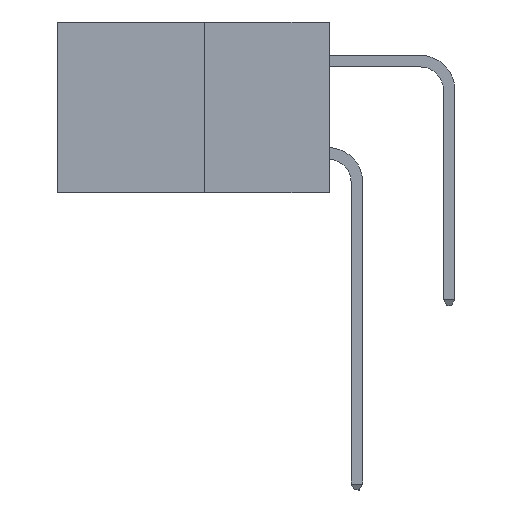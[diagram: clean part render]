
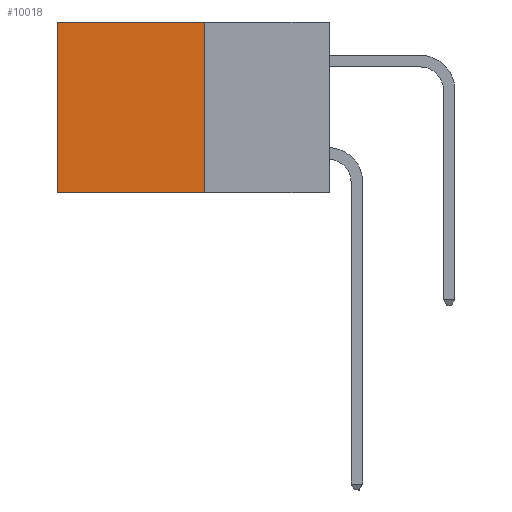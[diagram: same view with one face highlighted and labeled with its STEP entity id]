
A CAD part, left-side view. The second image highlights one B-rep face of the part: STEP entity #10018.
In plain terms, the highlighted planar face has unit normal (-1, 0, 0).
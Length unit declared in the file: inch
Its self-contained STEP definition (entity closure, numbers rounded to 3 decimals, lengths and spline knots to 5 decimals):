
#213 = ORIENTED_EDGE ( 'NONE', *, *, #5932, .T. ) ;
#272 = VECTOR ( 'NONE', #13073, 39.37008 ) ;
#283 = ORIENTED_EDGE ( 'NONE', *, *, #8095, .F. ) ;
#650 = VERTEX_POINT ( 'NONE', #18060 ) ;
#937 = ORIENTED_EDGE ( 'NONE', *, *, #4957, .F. ) ;
#2012 = VECTOR ( 'NONE', #16059, 39.37008 ) ;
#2642 = ORIENTED_EDGE ( 'NONE', *, *, #15275, .T. ) ;
#2751 = FACE_OUTER_BOUND ( 'NONE', #8653, .T. ) ;
#2906 = CARTESIAN_POINT ( 'NONE',  ( 0.277, 0.27, 0. ) ) ;
#4400 = PLANE ( 'NONE',  #9622 ) ;
#4454 = DIRECTION ( 'NONE',  ( 0., 0., -1. ) ) ;
#4722 = CARTESIAN_POINT ( 'NONE',  ( 0.277, 0.59, -0.37 ) ) ;
#4957 = EDGE_CURVE ( 'NONE', #17669, #8572, #16429, .T. ) ;
#5798 = DIRECTION ( 'NONE',  ( 0., 0., -1. ) ) ;
#5932 = EDGE_CURVE ( 'NONE', #11860, #650, #10958, .T. ) ;
#8095 = EDGE_CURVE ( 'NONE', #11860, #17669, #15264, .T. ) ;
#8271 = VECTOR ( 'NONE', #4454, 39.37008 ) ;
#8572 = VERTEX_POINT ( 'NONE', #17896 ) ;
#8653 = EDGE_LOOP ( 'NONE', ( #2642, #937, #283, #213 ) ) ;
#9010 = LINE ( 'NONE', #4722, #272 ) ;
#9176 = CARTESIAN_POINT ( 'NONE',  ( 0.277, 0.27, 0. ) ) ;
#9622 = AXIS2_PLACEMENT_3D ( 'NONE', #16898, #14138, #5798 ) ;
#10018 = ADVANCED_FACE ( 'NONE', ( #2751 ), #4400, .F. ) ;
#10517 = VECTOR ( 'NONE', #11271, 39.37008 ) ;
#10958 = LINE ( 'NONE', #2906, #10517 ) ;
#11271 = DIRECTION ( 'NONE',  ( 0., 1., 0. ) ) ;
#11860 = VERTEX_POINT ( 'NONE', #9176 ) ;
#13073 = DIRECTION ( 'NONE',  ( 0., 0., -1. ) ) ;
#14138 = DIRECTION ( 'NONE',  ( 1., 0., 0. ) ) ;
#14193 = CARTESIAN_POINT ( 'NONE',  ( 0.277, 0.27, -0.37 ) ) ;
#14478 = CARTESIAN_POINT ( 'NONE',  ( 0.277, 0.27, -0.37 ) ) ;
#14656 = CARTESIAN_POINT ( 'NONE',  ( 0.277, 0.27, -0.37 ) ) ;
#15264 = LINE ( 'NONE', #14193, #8271 ) ;
#15275 = EDGE_CURVE ( 'NONE', #650, #8572, #9010, .T. ) ;
#16059 = DIRECTION ( 'NONE',  ( 0., 1., 0. ) ) ;
#16429 = LINE ( 'NONE', #14656, #2012 ) ;
#16898 = CARTESIAN_POINT ( 'NONE',  ( 0.277, 0.27, -0.37 ) ) ;
#17669 = VERTEX_POINT ( 'NONE', #14478 ) ;
#17896 = CARTESIAN_POINT ( 'NONE',  ( 0.277, 0.59, -0.37 ) ) ;
#18060 = CARTESIAN_POINT ( 'NONE',  ( 0.277, 0.59, 0. ) ) ;
